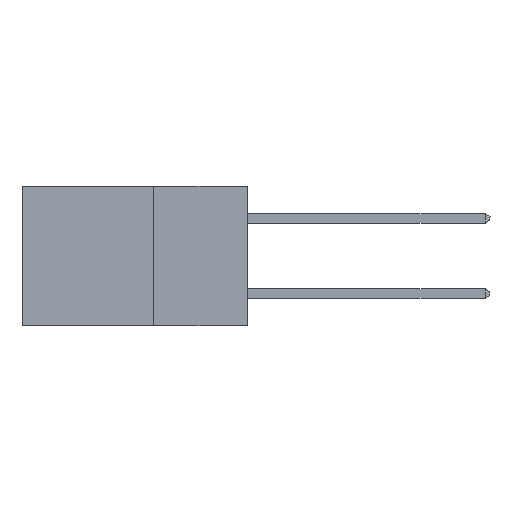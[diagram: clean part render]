
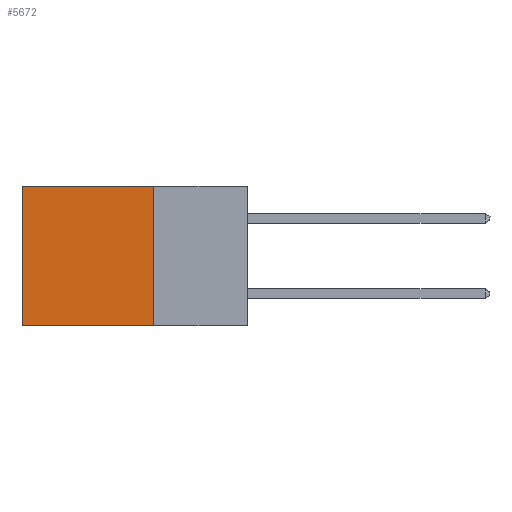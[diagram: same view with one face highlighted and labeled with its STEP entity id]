
A CAD part, left-side view. The second image highlights one B-rep face of the part: STEP entity #5672.
In plain terms, the highlighted planar face has unit normal (-1, 0, 0).
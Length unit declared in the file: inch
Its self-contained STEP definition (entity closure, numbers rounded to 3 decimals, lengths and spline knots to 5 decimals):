
#70 = VERTEX_POINT ( 'NONE', #5993 ) ;
#187 = EDGE_CURVE ( 'NONE', #4845, #4979, #7793, .T. ) ;
#263 = EDGE_CURVE ( 'NONE', #70, #4979, #1329, .T. ) ;
#297 = DIRECTION ( 'NONE',  ( 0., 1., 0. ) ) ;
#666 = LINE ( 'NONE', #6500, #3709 ) ;
#1329 = LINE ( 'NONE', #6546, #4840 ) ;
#1574 = VECTOR ( 'NONE', #9594, 39.37008 ) ;
#1990 = CARTESIAN_POINT ( 'NONE',  ( 0.2615, 0.25, -0.37 ) ) ;
#2020 = DIRECTION ( 'NONE',  ( 1., 0., 0. ) ) ;
#2337 = CARTESIAN_POINT ( 'NONE',  ( 0.2615, 0.25, 0. ) ) ;
#2718 = EDGE_CURVE ( 'NONE', #3783, #70, #9749, .T. ) ;
#3055 = CARTESIAN_POINT ( 'NONE',  ( 0.2615, 0.6, -0.37 ) ) ;
#3709 = VECTOR ( 'NONE', #9827, 39.37008 ) ;
#3783 = VERTEX_POINT ( 'NONE', #2337 ) ;
#4562 = ORIENTED_EDGE ( 'NONE', *, *, #11069, .F. ) ;
#4840 = VECTOR ( 'NONE', #9098, 39.37008 ) ;
#4845 = VERTEX_POINT ( 'NONE', #1990 ) ;
#4979 = VERTEX_POINT ( 'NONE', #3055 ) ;
#5672 = ADVANCED_FACE ( 'NONE', ( #8398 ), #9726, .F. ) ;
#5993 = CARTESIAN_POINT ( 'NONE',  ( 0.2615, 0.6, 0. ) ) ;
#6500 = CARTESIAN_POINT ( 'NONE',  ( 0.2615, 0.25, -0.37 ) ) ;
#6546 = CARTESIAN_POINT ( 'NONE',  ( 0.2615, 0.6, -0.37 ) ) ;
#6987 = CARTESIAN_POINT ( 'NONE',  ( 0.2615, 0.25, -0.37 ) ) ;
#7793 = LINE ( 'NONE', #6987, #1574 ) ;
#8004 = CARTESIAN_POINT ( 'NONE',  ( 0.2615, 0.25, 0. ) ) ;
#8398 = FACE_OUTER_BOUND ( 'NONE', #10927, .T. ) ;
#9098 = DIRECTION ( 'NONE',  ( 0., 0., -1. ) ) ;
#9500 = DIRECTION ( 'NONE',  ( 0., 0., -1. ) ) ;
#9594 = DIRECTION ( 'NONE',  ( 0., 1., 0. ) ) ;
#9660 = CARTESIAN_POINT ( 'NONE',  ( 0.2615, 0.25, -0.37 ) ) ;
#9726 = PLANE ( 'NONE',  #10086 ) ;
#9749 = LINE ( 'NONE', #8004, #10346 ) ;
#9827 = DIRECTION ( 'NONE',  ( 0., 0., -1. ) ) ;
#10086 = AXIS2_PLACEMENT_3D ( 'NONE', #9660, #2020, #9500 ) ;
#10138 = ORIENTED_EDGE ( 'NONE', *, *, #263, .T. ) ;
#10346 = VECTOR ( 'NONE', #297, 39.37008 ) ;
#10704 = ORIENTED_EDGE ( 'NONE', *, *, #2718, .T. ) ;
#10713 = ORIENTED_EDGE ( 'NONE', *, *, #187, .F. ) ;
#10927 = EDGE_LOOP ( 'NONE', ( #10138, #10713, #4562, #10704 ) ) ;
#11069 = EDGE_CURVE ( 'NONE', #3783, #4845, #666, .T. ) ;
